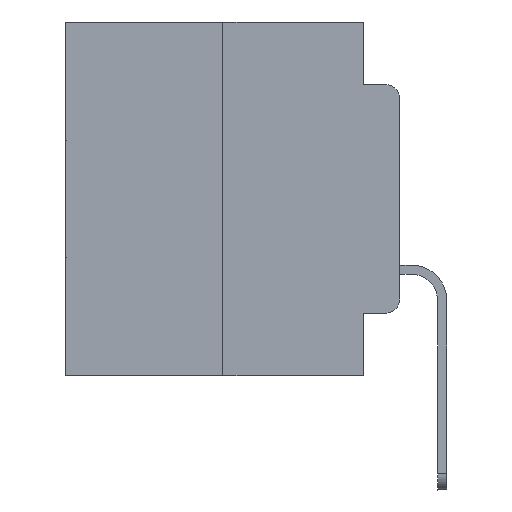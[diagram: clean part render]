
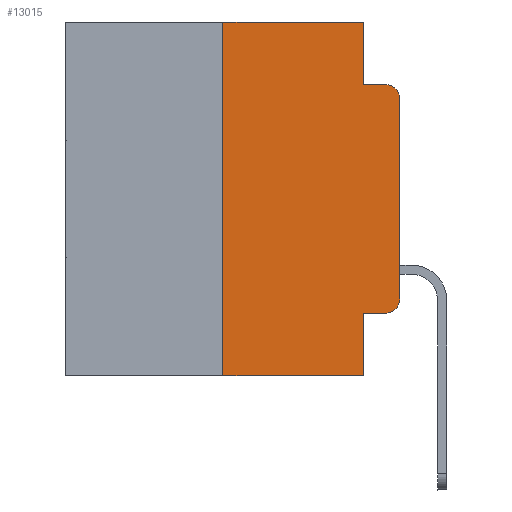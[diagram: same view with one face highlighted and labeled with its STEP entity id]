
A CAD part, left-side view. The second image highlights one B-rep face of the part: STEP entity #13015.
In plain terms, the highlighted planar face has unit normal (-1, 0, 0).
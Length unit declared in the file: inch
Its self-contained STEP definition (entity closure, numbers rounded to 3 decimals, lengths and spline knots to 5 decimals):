
#483 = CARTESIAN_POINT ( 'NONE',  ( 0., 0.02, -0.3915 ) ) ;
#982 = DIRECTION ( 'NONE',  ( 0., 0., -1. ) ) ;
#1301 = VECTOR ( 'NONE', #982, 39.37008 ) ;
#2228 = LINE ( 'NONE', #8528, #24590 ) ;
#2509 = FACE_OUTER_BOUND ( 'NONE', #5202, .T. ) ;
#2868 = LINE ( 'NONE', #21520, #25337 ) ;
#3405 = VERTEX_POINT ( 'NONE', #5244 ) ;
#3917 = CARTESIAN_POINT ( 'NONE',  ( 0., 0.051, -0.5 ) ) ;
#3918 = AXIS2_PLACEMENT_3D ( 'NONE', #25345, #16866, #23050 ) ;
#4010 = ORIENTED_EDGE ( 'NONE', *, *, #5723, .T. ) ;
#4254 = DIRECTION ( 'NONE',  ( 0., 0., -1. ) ) ;
#5202 = EDGE_LOOP ( 'NONE', ( #13192, #12284, #6778, #24180, #6982, #25416, #6215, #7732, #10414, #4010 ) ) ;
#5244 = CARTESIAN_POINT ( 'NONE',  ( 0., 0.051, 0. ) ) ;
#5723 = EDGE_CURVE ( 'NONE', #21067, #12501, #11860, .T. ) ;
#5938 = DIRECTION ( 'NONE',  ( 0., 0., -1. ) ) ;
#6215 = ORIENTED_EDGE ( 'NONE', *, *, #10299, .T. ) ;
#6778 = ORIENTED_EDGE ( 'NONE', *, *, #25024, .F. ) ;
#6982 = ORIENTED_EDGE ( 'NONE', *, *, #14315, .F. ) ;
#7270 = DIRECTION ( 'NONE',  ( 0., -1., 0. ) ) ;
#7332 = VERTEX_POINT ( 'NONE', #7842 ) ;
#7673 = EDGE_CURVE ( 'NONE', #3405, #7332, #23276, .T. ) ;
#7714 = VECTOR ( 'NONE', #25568, 39.37008 ) ;
#7732 = ORIENTED_EDGE ( 'NONE', *, *, #17975, .F. ) ;
#7842 = CARTESIAN_POINT ( 'NONE',  ( 0., 0.051, -0.0885 ) ) ;
#8528 = CARTESIAN_POINT ( 'NONE',  ( 0., 0.25, 0. ) ) ;
#8711 = CARTESIAN_POINT ( 'NONE',  ( 0., 0.051, -0.4115 ) ) ;
#8797 = EDGE_CURVE ( 'NONE', #20136, #21017, #26232, .T. ) ;
#9164 = CARTESIAN_POINT ( 'NONE',  ( 0., 0.051, -0.4115 ) ) ;
#9295 = VECTOR ( 'NONE', #7270, 39.37008 ) ;
#9297 = AXIS2_PLACEMENT_3D ( 'NONE', #483, #22906, #4254 ) ;
#10000 = LINE ( 'NONE', #16180, #15147 ) ;
#10175 = CARTESIAN_POINT ( 'NONE',  ( 0., 0.02, -0.1085 ) ) ;
#10284 = EDGE_CURVE ( 'NONE', #23592, #21067, #22740, .T. ) ;
#10299 = EDGE_CURVE ( 'NONE', #19096, #10579, #2868, .T. ) ;
#10414 = ORIENTED_EDGE ( 'NONE', *, *, #10284, .T. ) ;
#10579 = VERTEX_POINT ( 'NONE', #3917 ) ;
#10739 = CARTESIAN_POINT ( 'NONE',  ( 0., 0.02, -0.0885 ) ) ;
#10960 = PLANE ( 'NONE',  #3918 ) ;
#11051 = DIRECTION ( 'NONE',  ( 0., -1., 0. ) ) ;
#11120 = CARTESIAN_POINT ( 'NONE',  ( 0., 0., -0.3915 ) ) ;
#11614 = AXIS2_PLACEMENT_3D ( 'NONE', #10175, #12304, #20768 ) ;
#11860 = CIRCLE ( 'NONE', #9297, 0.02 ) ;
#11901 = LINE ( 'NONE', #20224, #25244 ) ;
#12284 = ORIENTED_EDGE ( 'NONE', *, *, #8797, .T. ) ;
#12304 = DIRECTION ( 'NONE',  ( -1., 0., 0. ) ) ;
#12501 = VERTEX_POINT ( 'NONE', #11120 ) ;
#13015 = ADVANCED_FACE ( 'NONE', ( #2509 ), #10960, .F. ) ;
#13058 = CARTESIAN_POINT ( 'NONE',  ( 0., 0.051, 0. ) ) ;
#13192 = ORIENTED_EDGE ( 'NONE', *, *, #26348, .T. ) ;
#13560 = CARTESIAN_POINT ( 'NONE',  ( 0., 0.051, -0.0885 ) ) ;
#13598 = VERTEX_POINT ( 'NONE', #16493 ) ;
#14315 = EDGE_CURVE ( 'NONE', #13598, #3405, #10000, .T. ) ;
#14915 = CARTESIAN_POINT ( 'NONE',  ( 0., 0.02, -0.4115 ) ) ;
#15147 = VECTOR ( 'NONE', #24377, 39.37008 ) ;
#16180 = CARTESIAN_POINT ( 'NONE',  ( 0., 0.473, 0. ) ) ;
#16493 = CARTESIAN_POINT ( 'NONE',  ( 0., 0.25, 0. ) ) ;
#16866 = DIRECTION ( 'NONE',  ( 1., 0., 0. ) ) ;
#16956 = EDGE_CURVE ( 'NONE', #19096, #13598, #2228, .T. ) ;
#17975 = EDGE_CURVE ( 'NONE', #23592, #10579, #21790, .T. ) ;
#18596 = DIRECTION ( 'NONE',  ( 0., 0., 1. ) ) ;
#18626 = CARTESIAN_POINT ( 'NONE',  ( 0., 0., -0.1085 ) ) ;
#19096 = VERTEX_POINT ( 'NONE', #19113 ) ;
#19113 = CARTESIAN_POINT ( 'NONE',  ( 0., 0.25, -0.5 ) ) ;
#20136 = VERTEX_POINT ( 'NONE', #18626 ) ;
#20224 = CARTESIAN_POINT ( 'NONE',  ( 0., 0., 0. ) ) ;
#20335 = VECTOR ( 'NONE', #5938, 39.37008 ) ;
#20768 = DIRECTION ( 'NONE',  ( 0., 0., -1. ) ) ;
#21017 = VERTEX_POINT ( 'NONE', #10739 ) ;
#21067 = VERTEX_POINT ( 'NONE', #14915 ) ;
#21520 = CARTESIAN_POINT ( 'NONE',  ( 0., 0.473, -0.5 ) ) ;
#21790 = LINE ( 'NONE', #22047, #20335 ) ;
#22047 = CARTESIAN_POINT ( 'NONE',  ( 0., 0.051, 0. ) ) ;
#22740 = LINE ( 'NONE', #9164, #7714 ) ;
#22906 = DIRECTION ( 'NONE',  ( -1., 0., 0. ) ) ;
#23050 = DIRECTION ( 'NONE',  ( 0., 0., -1. ) ) ;
#23276 = LINE ( 'NONE', #13058, #1301 ) ;
#23592 = VERTEX_POINT ( 'NONE', #8711 ) ;
#24180 = ORIENTED_EDGE ( 'NONE', *, *, #7673, .F. ) ;
#24260 = DIRECTION ( 'NONE',  ( 0., 0., 1. ) ) ;
#24377 = DIRECTION ( 'NONE',  ( 0., -1., 0. ) ) ;
#24590 = VECTOR ( 'NONE', #18596, 39.37008 ) ;
#25024 = EDGE_CURVE ( 'NONE', #7332, #21017, #25946, .T. ) ;
#25244 = VECTOR ( 'NONE', #24260, 39.37008 ) ;
#25337 = VECTOR ( 'NONE', #11051, 39.37008 ) ;
#25345 = CARTESIAN_POINT ( 'NONE',  ( 0., 0.473, 0. ) ) ;
#25416 = ORIENTED_EDGE ( 'NONE', *, *, #16956, .F. ) ;
#25568 = DIRECTION ( 'NONE',  ( 0., -1., 0. ) ) ;
#25946 = LINE ( 'NONE', #13560, #9295 ) ;
#26232 = CIRCLE ( 'NONE', #11614, 0.02 ) ;
#26348 = EDGE_CURVE ( 'NONE', #12501, #20136, #11901, .T. ) ;
